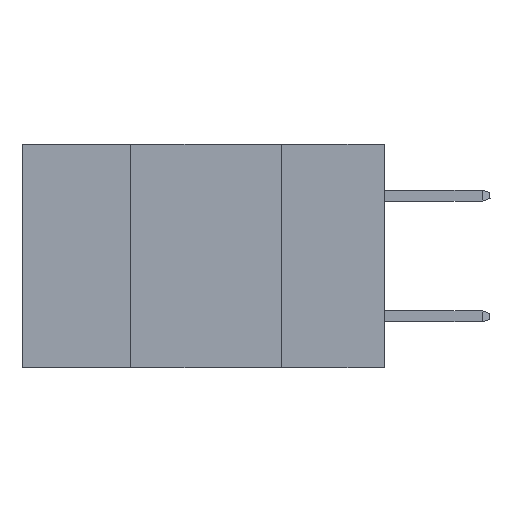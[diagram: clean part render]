
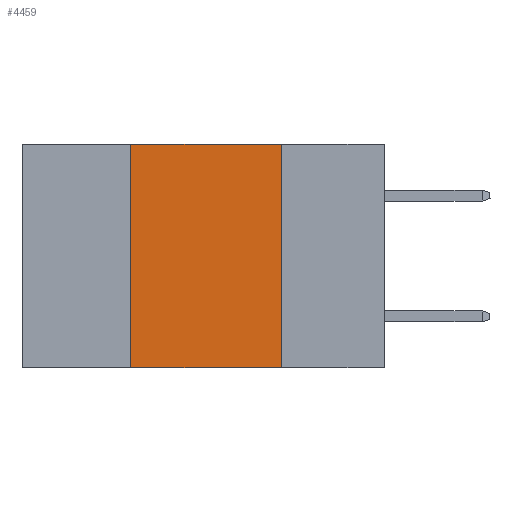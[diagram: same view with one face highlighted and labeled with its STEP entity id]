
A CAD part, left-side view. The second image highlights one B-rep face of the part: STEP entity #4459.
In plain terms, the highlighted planar face has unit normal (-1, 0, 0).
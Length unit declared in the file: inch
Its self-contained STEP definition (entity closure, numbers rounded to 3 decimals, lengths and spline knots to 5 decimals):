
#452 = PLANE ( 'NONE',  #1645 ) ;
#779 = DIRECTION ( 'NONE',  ( 0., -1., 0. ) ) ;
#1203 = EDGE_CURVE ( 'NONE', #5992, #17024, #6947, .T. ) ;
#1253 = DIRECTION ( 'NONE',  ( 0., -1., 0. ) ) ;
#1559 = CARTESIAN_POINT ( 'NONE',  ( 0., 0.42, -0.37 ) ) ;
#1645 = AXIS2_PLACEMENT_3D ( 'NONE', #10373, #2374, #12076 ) ;
#2163 = VECTOR ( 'NONE', #7864, 39.37008 ) ;
#2290 = LINE ( 'NONE', #14860, #5939 ) ;
#2374 = DIRECTION ( 'NONE',  ( 1., 0., 0. ) ) ;
#3652 = CARTESIAN_POINT ( 'NONE',  ( 0., 0.17, 0. ) ) ;
#3879 = LINE ( 'NONE', #3652, #2163 ) ;
#4366 = EDGE_CURVE ( 'NONE', #17024, #16323, #2290, .T. ) ;
#4459 = ADVANCED_FACE ( 'NONE', ( #12905 ), #452, .F. ) ;
#4462 = VECTOR ( 'NONE', #1253, 39.37008 ) ;
#4623 = DIRECTION ( 'NONE',  ( 0., 0., 1. ) ) ;
#5340 = ORIENTED_EDGE ( 'NONE', *, *, #7425, .T. ) ;
#5575 = VERTEX_POINT ( 'NONE', #15562 ) ;
#5939 = VECTOR ( 'NONE', #779, 39.37008 ) ;
#5992 = VERTEX_POINT ( 'NONE', #1559 ) ;
#6947 = LINE ( 'NONE', #17036, #9794 ) ;
#6948 = CARTESIAN_POINT ( 'NONE',  ( 0., 0.17, 0. ) ) ;
#7425 = EDGE_CURVE ( 'NONE', #5992, #5575, #14308, .T. ) ;
#7864 = DIRECTION ( 'NONE',  ( 0., 0., -1. ) ) ;
#8191 = CARTESIAN_POINT ( 'NONE',  ( 0., 0.6, -0.37 ) ) ;
#9794 = VECTOR ( 'NONE', #4623, 39.37008 ) ;
#10373 = CARTESIAN_POINT ( 'NONE',  ( 0., 0.6, 0. ) ) ;
#10503 = ORIENTED_EDGE ( 'NONE', *, *, #4366, .F. ) ;
#10900 = EDGE_LOOP ( 'NONE', ( #14670, #10503, #16467, #5340 ) ) ;
#12076 = DIRECTION ( 'NONE',  ( 0., 0., -1. ) ) ;
#12905 = FACE_OUTER_BOUND ( 'NONE', #10900, .T. ) ;
#14308 = LINE ( 'NONE', #8191, #4462 ) ;
#14670 = ORIENTED_EDGE ( 'NONE', *, *, #14835, .F. ) ;
#14835 = EDGE_CURVE ( 'NONE', #16323, #5575, #3879, .T. ) ;
#14860 = CARTESIAN_POINT ( 'NONE',  ( 0., 0.6, 0. ) ) ;
#15562 = CARTESIAN_POINT ( 'NONE',  ( 0., 0.17, -0.37 ) ) ;
#16323 = VERTEX_POINT ( 'NONE', #6948 ) ;
#16467 = ORIENTED_EDGE ( 'NONE', *, *, #1203, .F. ) ;
#17024 = VERTEX_POINT ( 'NONE', #17863 ) ;
#17036 = CARTESIAN_POINT ( 'NONE',  ( 0., 0.42, 0. ) ) ;
#17863 = CARTESIAN_POINT ( 'NONE',  ( 0., 0.42, 0. ) ) ;
